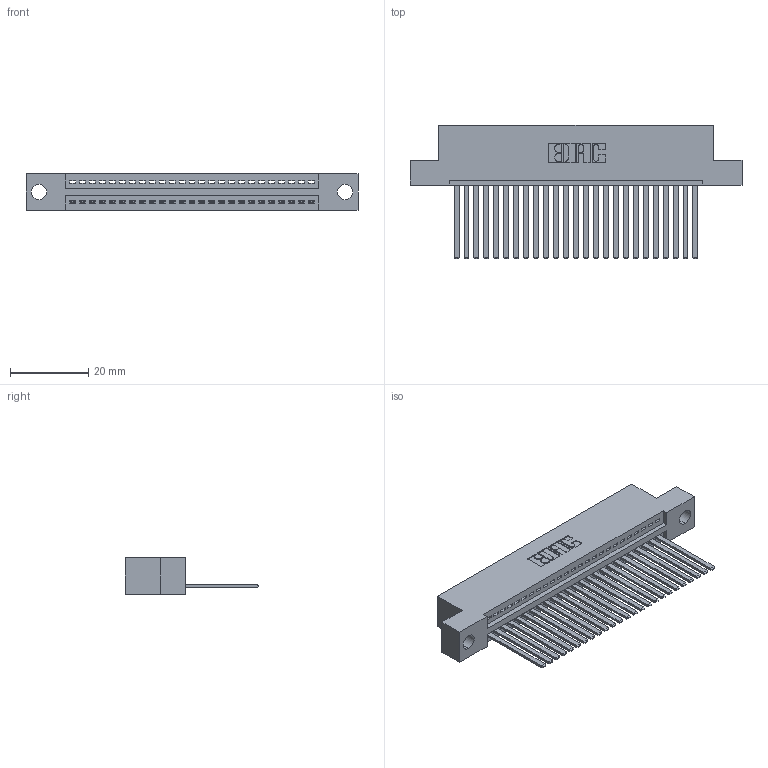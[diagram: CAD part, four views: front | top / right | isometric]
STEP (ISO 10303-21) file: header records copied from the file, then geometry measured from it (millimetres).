
FILE_DESCRIPTION (( 'STEP AP203' ), '1' );
FILE_NAME ('345-025-544-104.STEP', '2019-10-05T07:33:12', ( '' ), ( '' ), 'SwSTEP 2.0', 'SolidWorks 2016', '' );
FILE_SCHEMA (( 'CONFIG_CONTROL_DESIGN' ));
Length unit declared in the file: inch
Products named in the file (3): 345-025-544-104; 345 Part_Flush Mounting Lugs - 0.156 Dia-TH; 345-292-001_345-293-144
Assembly tree (26 placements, depth 2):
  345-025-544-104
    345 Part_Flush Mounting Lugs - 0.156 Dia-TH
    345-292-001_345-293-144  x25
Bounding box: 84.71 x 33.96 x 9.4 mm (x, y, z)
Volume: 8108.2 mm3; surface area: 11221.9 mm2
Topology: 26 solids, 26 shells, 1426 faces, 4291 edges, 2826 vertices
Faces by surface type: plane 980, cylinder 446
Entity records: 20923 total; most frequent: CARTESIAN_POINT 3631, ORIENTED_EDGE 3590, DIRECTION 3193, EDGE_CURVE 1795, LINE 1567, VECTOR 1567, VERTEX_POINT 1194, AXIS2_PLACEMENT_3D 813
